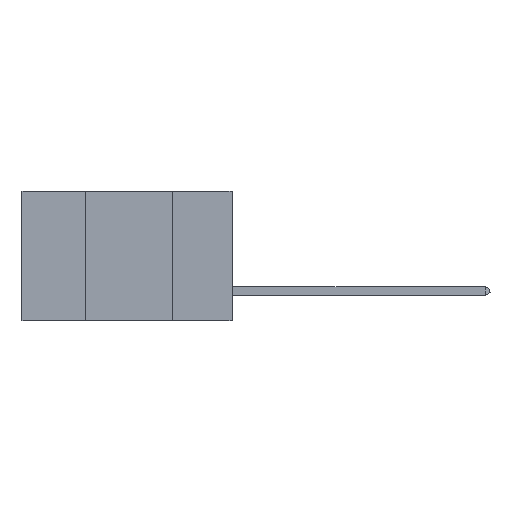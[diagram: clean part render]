
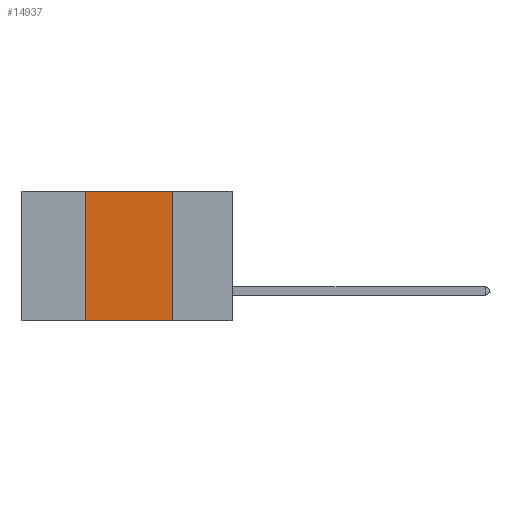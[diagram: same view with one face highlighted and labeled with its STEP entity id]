
A CAD part, left-side view. The second image highlights one B-rep face of the part: STEP entity #14937.
In plain terms, the highlighted planar face has unit normal (-1, 0, 0).
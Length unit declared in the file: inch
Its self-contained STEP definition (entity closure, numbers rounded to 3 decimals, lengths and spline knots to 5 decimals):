
#40 = VECTOR ( 'NONE', #14616, 39.37008 ) ;
#178 = PLANE ( 'NONE',  #9710 ) ;
#618 = DIRECTION ( 'NONE',  ( 0., -1., 0. ) ) ;
#1809 = DIRECTION ( 'NONE',  ( 1., 0., 0. ) ) ;
#2636 = EDGE_LOOP ( 'NONE', ( #7555, #8185, #19309, #16021 ) ) ;
#3520 = VERTEX_POINT ( 'NONE', #17390 ) ;
#3905 = EDGE_CURVE ( 'NONE', #3520, #19476, #9550, .T. ) ;
#4133 = VECTOR ( 'NONE', #4896, 39.37008 ) ;
#4896 = DIRECTION ( 'NONE',  ( 0., 0., -1. ) ) ;
#5437 = CARTESIAN_POINT ( 'NONE',  ( 0., 0.42, 0. ) ) ;
#5866 = EDGE_CURVE ( 'NONE', #8936, #9959, #9455, .T. ) ;
#6375 = DIRECTION ( 'NONE',  ( 0., 0., -1. ) ) ;
#7555 = ORIENTED_EDGE ( 'NONE', *, *, #17884, .F. ) ;
#7989 = CARTESIAN_POINT ( 'NONE',  ( 0., 0.17, 0. ) ) ;
#8185 = ORIENTED_EDGE ( 'NONE', *, *, #5866, .F. ) ;
#8199 = LINE ( 'NONE', #7989, #4133 ) ;
#8936 = VERTEX_POINT ( 'NONE', #5437 ) ;
#9455 = LINE ( 'NONE', #14241, #18572 ) ;
#9550 = LINE ( 'NONE', #14422, #40 ) ;
#9710 = AXIS2_PLACEMENT_3D ( 'NONE', #17041, #1809, #6375 ) ;
#9959 = VERTEX_POINT ( 'NONE', #13913 ) ;
#9980 = CARTESIAN_POINT ( 'NONE',  ( 0., 0.17, -0.37 ) ) ;
#10200 = DIRECTION ( 'NONE',  ( 0., 0., 1. ) ) ;
#11157 = EDGE_CURVE ( 'NONE', #3520, #8936, #19512, .T. ) ;
#13913 = CARTESIAN_POINT ( 'NONE',  ( 0., 0.17, 0. ) ) ;
#14241 = CARTESIAN_POINT ( 'NONE',  ( 0., 0.6, 0. ) ) ;
#14245 = FACE_OUTER_BOUND ( 'NONE', #2636, .T. ) ;
#14422 = CARTESIAN_POINT ( 'NONE',  ( 0., 0.6, -0.37 ) ) ;
#14616 = DIRECTION ( 'NONE',  ( 0., -1., 0. ) ) ;
#14937 = ADVANCED_FACE ( 'NONE', ( #14245 ), #178, .F. ) ;
#15876 = VECTOR ( 'NONE', #10200, 39.37008 ) ;
#16021 = ORIENTED_EDGE ( 'NONE', *, *, #3905, .T. ) ;
#16258 = CARTESIAN_POINT ( 'NONE',  ( 0., 0.42, 0. ) ) ;
#17041 = CARTESIAN_POINT ( 'NONE',  ( 0., 0.6, 0. ) ) ;
#17390 = CARTESIAN_POINT ( 'NONE',  ( 0., 0.42, -0.37 ) ) ;
#17884 = EDGE_CURVE ( 'NONE', #9959, #19476, #8199, .T. ) ;
#18572 = VECTOR ( 'NONE', #618, 39.37008 ) ;
#19309 = ORIENTED_EDGE ( 'NONE', *, *, #11157, .F. ) ;
#19476 = VERTEX_POINT ( 'NONE', #9980 ) ;
#19512 = LINE ( 'NONE', #16258, #15876 ) ;
